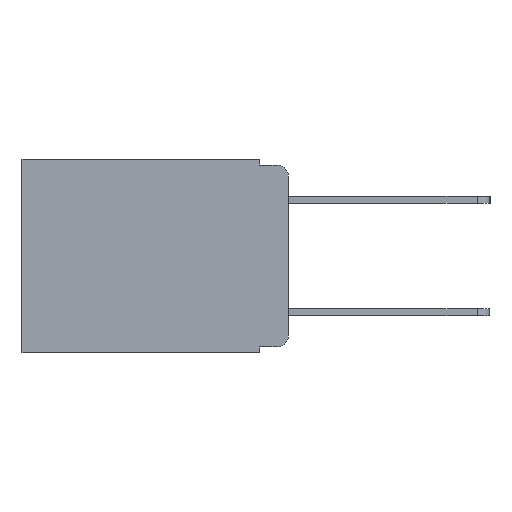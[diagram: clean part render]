
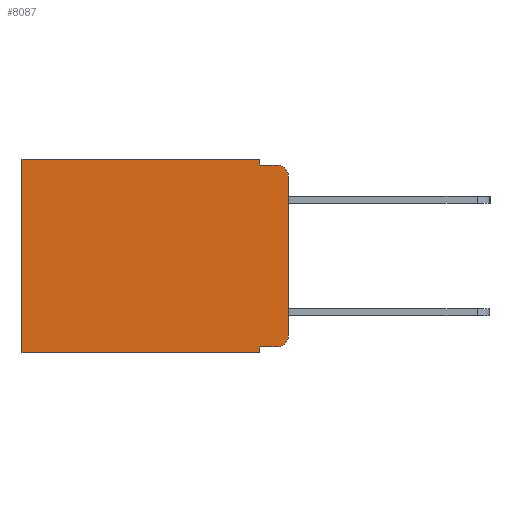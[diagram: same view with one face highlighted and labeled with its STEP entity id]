
A CAD part, left-side view. The second image highlights one B-rep face of the part: STEP entity #8087.
In plain terms, the highlighted planar face has unit normal (-1, 0, 0).
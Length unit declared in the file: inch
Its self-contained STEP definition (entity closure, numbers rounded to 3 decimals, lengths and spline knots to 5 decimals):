
#747 = VERTEX_POINT ( 'NONE', #15084 ) ;
#833 = VERTEX_POINT ( 'NONE', #5914 ) ;
#1081 = ORIENTED_EDGE ( 'NONE', *, *, #5941, .T. ) ;
#1193 = DIRECTION ( 'NONE',  ( 0., -1., 0. ) ) ;
#1511 = DIRECTION ( 'NONE',  ( 0., 0., -1. ) ) ;
#1574 = LINE ( 'NONE', #9581, #10961 ) ;
#1632 = ORIENTED_EDGE ( 'NONE', *, *, #16213, .T. ) ;
#1756 = EDGE_CURVE ( 'NONE', #11019, #8404, #14884, .T. ) ;
#2156 = AXIS2_PLACEMENT_3D ( 'NONE', #18558, #8719, #20184 ) ;
#2327 = CARTESIAN_POINT ( 'NONE',  ( 0.298, 0., 0. ) ) ;
#2428 = ORIENTED_EDGE ( 'NONE', *, *, #5810, .T. ) ;
#2798 = DIRECTION ( 'NONE',  ( -1., 0., 0. ) ) ;
#2978 = EDGE_LOOP ( 'NONE', ( #19133, #1081, #6775, #8089, #3172, #4978, #19411, #18937, #1632, #2428 ) ) ;
#3051 = CARTESIAN_POINT ( 'NONE',  ( 0.298, 0.051, 0. ) ) ;
#3172 = ORIENTED_EDGE ( 'NONE', *, *, #1756, .T. ) ;
#3840 = CARTESIAN_POINT ( 'NONE',  ( 0.298, 0.02, -0.01 ) ) ;
#3887 = AXIS2_PLACEMENT_3D ( 'NONE', #21222, #11481, #1511 ) ;
#4699 = DIRECTION ( 'NONE',  ( 0., 0., -1. ) ) ;
#4978 = ORIENTED_EDGE ( 'NONE', *, *, #8860, .T. ) ;
#5190 = VERTEX_POINT ( 'NONE', #19305 ) ;
#5366 = PLANE ( 'NONE',  #2156 ) ;
#5630 = CARTESIAN_POINT ( 'NONE',  ( 0.298, 0.051, -0.333 ) ) ;
#5723 = LINE ( 'NONE', #20296, #18359 ) ;
#5810 = EDGE_CURVE ( 'NONE', #12685, #13595, #20653, .T. ) ;
#5874 = EDGE_CURVE ( 'NONE', #747, #13595, #1574, .T. ) ;
#5914 = CARTESIAN_POINT ( 'NONE',  ( 0.298, 0.051, -0.01 ) ) ;
#5941 = EDGE_CURVE ( 'NONE', #747, #14177, #17620, .T. ) ;
#6770 = DIRECTION ( 'NONE',  ( 0., 0., -1. ) ) ;
#6775 = ORIENTED_EDGE ( 'NONE', *, *, #17007, .F. ) ;
#8087 = ADVANCED_FACE ( 'NONE', ( #10085 ), #5366, .F. ) ;
#8089 = ORIENTED_EDGE ( 'NONE', *, *, #21307, .F. ) ;
#8404 = VERTEX_POINT ( 'NONE', #11873 ) ;
#8719 = DIRECTION ( 'NONE',  ( 1., 0., 0. ) ) ;
#8860 = EDGE_CURVE ( 'NONE', #8404, #14075, #5723, .T. ) ;
#9581 = CARTESIAN_POINT ( 'NONE',  ( 0.298, 0., 0. ) ) ;
#10085 = FACE_OUTER_BOUND ( 'NONE', #2978, .T. ) ;
#10482 = VECTOR ( 'NONE', #17024, 39.37008 ) ;
#10961 = VECTOR ( 'NONE', #21021, 39.37008 ) ;
#10986 = AXIS2_PLACEMENT_3D ( 'NONE', #12717, #2798, #14376 ) ;
#11019 = VERTEX_POINT ( 'NONE', #16677 ) ;
#11322 = LINE ( 'NONE', #3051, #15178 ) ;
#11374 = DIRECTION ( 'NONE',  ( 0., 1., 0. ) ) ;
#11481 = DIRECTION ( 'NONE',  ( -1., 0., 0. ) ) ;
#11804 = CARTESIAN_POINT ( 'NONE',  ( 0.298, 0.051, 0. ) ) ;
#11873 = CARTESIAN_POINT ( 'NONE',  ( 0.298, 0.473, 0. ) ) ;
#12051 = VECTOR ( 'NONE', #6770, 39.37008 ) ;
#12072 = VECTOR ( 'NONE', #15538, 39.37008 ) ;
#12201 = EDGE_CURVE ( 'NONE', #15021, #5190, #11322, .T. ) ;
#12685 = VERTEX_POINT ( 'NONE', #17527 ) ;
#12717 = CARTESIAN_POINT ( 'NONE',  ( 0.298, 0.02, -0.313 ) ) ;
#13487 = CARTESIAN_POINT ( 'NONE',  ( 0.298, 0.473, -0.343 ) ) ;
#13595 = VERTEX_POINT ( 'NONE', #16727 ) ;
#13858 = DIRECTION ( 'NONE',  ( 0., 0., -1. ) ) ;
#14075 = VERTEX_POINT ( 'NONE', #13487 ) ;
#14177 = VERTEX_POINT ( 'NONE', #3840 ) ;
#14376 = DIRECTION ( 'NONE',  ( 0., 0., -1. ) ) ;
#14617 = VECTOR ( 'NONE', #1193, 39.37008 ) ;
#14884 = LINE ( 'NONE', #2327, #10482 ) ;
#15021 = VERTEX_POINT ( 'NONE', #17377 ) ;
#15084 = CARTESIAN_POINT ( 'NONE',  ( 0.298, 0., -0.03 ) ) ;
#15178 = VECTOR ( 'NONE', #4699, 39.37008 ) ;
#15538 = DIRECTION ( 'NONE',  ( 0., -1., 0. ) ) ;
#16030 = CARTESIAN_POINT ( 'NONE',  ( 0.298, 0.051, -0.01 ) ) ;
#16213 = EDGE_CURVE ( 'NONE', #15021, #12685, #21219, .T. ) ;
#16601 = EDGE_CURVE ( 'NONE', #5190, #14075, #18450, .T. ) ;
#16677 = CARTESIAN_POINT ( 'NONE',  ( 0.298, 0.051, 0. ) ) ;
#16727 = CARTESIAN_POINT ( 'NONE',  ( 0.298, 0., -0.313 ) ) ;
#17007 = EDGE_CURVE ( 'NONE', #833, #14177, #18950, .T. ) ;
#17024 = DIRECTION ( 'NONE',  ( 0., 1., 0. ) ) ;
#17377 = CARTESIAN_POINT ( 'NONE',  ( 0.298, 0.051, -0.333 ) ) ;
#17527 = CARTESIAN_POINT ( 'NONE',  ( 0.298, 0.02, -0.333 ) ) ;
#17620 = CIRCLE ( 'NONE', #3887, 0.02 ) ;
#17945 = VECTOR ( 'NONE', #11374, 39.37008 ) ;
#18359 = VECTOR ( 'NONE', #13858, 39.37008 ) ;
#18450 = LINE ( 'NONE', #19509, #17945 ) ;
#18558 = CARTESIAN_POINT ( 'NONE',  ( 0.298, 0., 0. ) ) ;
#18937 = ORIENTED_EDGE ( 'NONE', *, *, #12201, .F. ) ;
#18950 = LINE ( 'NONE', #16030, #14617 ) ;
#19133 = ORIENTED_EDGE ( 'NONE', *, *, #5874, .F. ) ;
#19305 = CARTESIAN_POINT ( 'NONE',  ( 0.298, 0.051, -0.343 ) ) ;
#19411 = ORIENTED_EDGE ( 'NONE', *, *, #16601, .F. ) ;
#19509 = CARTESIAN_POINT ( 'NONE',  ( 0.298, 0., -0.343 ) ) ;
#20184 = DIRECTION ( 'NONE',  ( 0., 0., -1. ) ) ;
#20296 = CARTESIAN_POINT ( 'NONE',  ( 0.298, 0.473, 0. ) ) ;
#20653 = CIRCLE ( 'NONE', #10986, 0.02 ) ;
#21021 = DIRECTION ( 'NONE',  ( 0., 0., -1. ) ) ;
#21202 = LINE ( 'NONE', #11804, #12051 ) ;
#21219 = LINE ( 'NONE', #5630, #12072 ) ;
#21222 = CARTESIAN_POINT ( 'NONE',  ( 0.298, 0.02, -0.03 ) ) ;
#21307 = EDGE_CURVE ( 'NONE', #11019, #833, #21202, .T. ) ;
